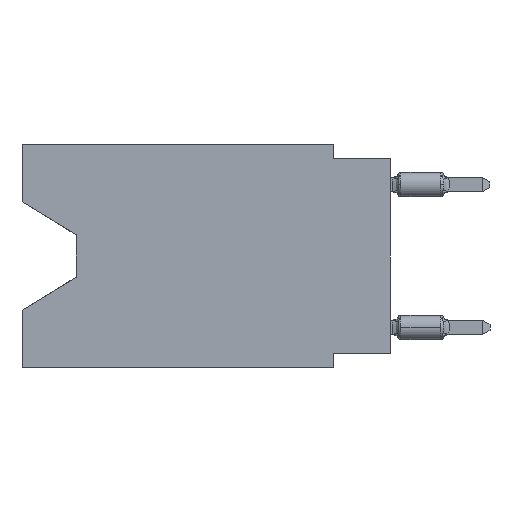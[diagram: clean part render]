
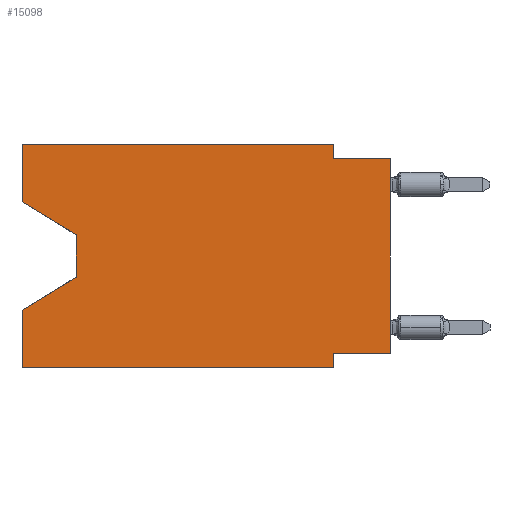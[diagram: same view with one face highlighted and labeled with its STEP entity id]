
A CAD part, left-side view. The second image highlights one B-rep face of the part: STEP entity #15098.
In plain terms, the highlighted planar face has unit normal (-1, 0, 0).
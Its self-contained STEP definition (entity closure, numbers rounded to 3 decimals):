
#19 = CARTESIAN_POINT ( 'NONE',  ( 0., 0., 0. ) ) ;
#44 = EDGE_LOOP ( 'NONE', ( #9401, #10544, #11426, #8220, #8632, #4534, #13998, #9303, #6205, #1182, #1276, #12741 ) ) ;
#261 = CARTESIAN_POINT ( 'NONE',  ( 0., 16.383, -7.36 ) ) ;
#678 = EDGE_CURVE ( 'NONE', #10650, #6573, #16260, .T. ) ;
#911 = VECTOR ( 'NONE', #5803, 1000. ) ;
#1005 = DIRECTION ( 'NONE',  ( 0., 0., -1. ) ) ;
#1182 = ORIENTED_EDGE ( 'NONE', *, *, #10891, .F. ) ;
#1225 = AXIS2_PLACEMENT_3D ( 'NONE', #1254, #7778, #1005 ) ;
#1254 = CARTESIAN_POINT ( 'NONE',  ( 0., 16.383, 0. ) ) ;
#1276 = ORIENTED_EDGE ( 'NONE', *, *, #12093, .F. ) ;
#1314 = CARTESIAN_POINT ( 'NONE',  ( 0., 16.383, 0. ) ) ;
#1611 = LINE ( 'NONE', #9928, #1913 ) ;
#1913 = VECTOR ( 'NONE', #12980, 1000. ) ;
#2863 = VECTOR ( 'NONE', #7139, 1000. ) ;
#2887 = VERTEX_POINT ( 'NONE', #13137 ) ;
#2916 = VECTOR ( 'NONE', #14248, 1000. ) ;
#4529 = CARTESIAN_POINT ( 'NONE',  ( 0., 2.54, 0. ) ) ;
#4534 = ORIENTED_EDGE ( 'NONE', *, *, #13500, .F. ) ;
#5208 = CARTESIAN_POINT ( 'NONE',  ( 0., 16.383, 0. ) ) ;
#5517 = VERTEX_POINT ( 'NONE', #261 ) ;
#5581 = CARTESIAN_POINT ( 'NONE',  ( 0., 16.383, -2.546 ) ) ;
#5620 = DIRECTION ( 'NONE',  ( 0., 0., -1. ) ) ;
#5654 = CARTESIAN_POINT ( 'NONE',  ( 0., 2.54, -9.271 ) ) ;
#5803 = DIRECTION ( 'NONE',  ( 0., 1., 0. ) ) ;
#5956 = VECTOR ( 'NONE', #5620, 1000. ) ;
#5979 = CARTESIAN_POINT ( 'NONE',  ( 0., 16.383, -2.546 ) ) ;
#6205 = ORIENTED_EDGE ( 'NONE', *, *, #11991, .F. ) ;
#6573 = VERTEX_POINT ( 'NONE', #11096 ) ;
#6591 = DIRECTION ( 'NONE',  ( 0., 0., -1. ) ) ;
#6621 = DIRECTION ( 'NONE',  ( 0., -1., 0. ) ) ;
#6687 = LINE ( 'NONE', #12307, #15581 ) ;
#7030 = CARTESIAN_POINT ( 'NONE',  ( 0., 0., -9.271 ) ) ;
#7057 = VECTOR ( 'NONE', #14948, 1000. ) ;
#7139 = DIRECTION ( 'NONE',  ( 0., 0., -1. ) ) ;
#7435 = VERTEX_POINT ( 'NONE', #4529 ) ;
#7647 = CARTESIAN_POINT ( 'NONE',  ( 0., 16.383, -9.906 ) ) ;
#7697 = VECTOR ( 'NONE', #13743, 1000. ) ;
#7778 = DIRECTION ( 'NONE',  ( 1., 0., 0. ) ) ;
#8040 = PLANE ( 'NONE',  #1225 ) ;
#8220 = ORIENTED_EDGE ( 'NONE', *, *, #9516, .F. ) ;
#8400 = VERTEX_POINT ( 'NONE', #12094 ) ;
#8482 = DIRECTION ( 'NONE',  ( 0., -0.855, -0.519 ) ) ;
#8632 = ORIENTED_EDGE ( 'NONE', *, *, #10677, .T. ) ;
#8814 = VECTOR ( 'NONE', #6621, 1000. ) ;
#9027 = CARTESIAN_POINT ( 'NONE',  ( 0., 2.54, -0.635 ) ) ;
#9072 = LINE ( 'NONE', #5208, #11628 ) ;
#9150 = LINE ( 'NONE', #7647, #2916 ) ;
#9303 = ORIENTED_EDGE ( 'NONE', *, *, #16847, .T. ) ;
#9354 = VECTOR ( 'NONE', #8482, 1000. ) ;
#9401 = ORIENTED_EDGE ( 'NONE', *, *, #13070, .T. ) ;
#9516 = EDGE_CURVE ( 'NONE', #12317, #5517, #1611, .T. ) ;
#9762 = CARTESIAN_POINT ( 'NONE',  ( 0., 13.97, -4.013 ) ) ;
#9928 = CARTESIAN_POINT ( 'NONE',  ( 0., 16.383, 0. ) ) ;
#10223 = LINE ( 'NONE', #11801, #8814 ) ;
#10544 = ORIENTED_EDGE ( 'NONE', *, *, #13833, .T. ) ;
#10650 = VERTEX_POINT ( 'NONE', #5979 ) ;
#10677 = EDGE_CURVE ( 'NONE', #12317, #8400, #9150, .T. ) ;
#10820 = VECTOR ( 'NONE', #13360, 1000. ) ;
#10891 = EDGE_CURVE ( 'NONE', #7435, #12380, #6687, .T. ) ;
#11096 = CARTESIAN_POINT ( 'NONE',  ( 0., 16.383, 0. ) ) ;
#11426 = ORIENTED_EDGE ( 'NONE', *, *, #15208, .T. ) ;
#11628 = VECTOR ( 'NONE', #14438, 1000. ) ;
#11801 = CARTESIAN_POINT ( 'NONE',  ( 0., 0., -0.635 ) ) ;
#11851 = VERTEX_POINT ( 'NONE', #5654 ) ;
#11991 = EDGE_CURVE ( 'NONE', #12380, #16071, #10223, .T. ) ;
#12093 = EDGE_CURVE ( 'NONE', #6573, #7435, #9072, .T. ) ;
#12094 = CARTESIAN_POINT ( 'NONE',  ( 0., 2.54, -9.906 ) ) ;
#12207 = CARTESIAN_POINT ( 'NONE',  ( 0., 0., -0.635 ) ) ;
#12307 = CARTESIAN_POINT ( 'NONE',  ( 0., 2.54, 0. ) ) ;
#12317 = VERTEX_POINT ( 'NONE', #12585 ) ;
#12336 = CARTESIAN_POINT ( 'NONE',  ( 0., 13.97, -5.893 ) ) ;
#12380 = VERTEX_POINT ( 'NONE', #9027 ) ;
#12414 = LINE ( 'NONE', #13569, #7697 ) ;
#12480 = LINE ( 'NONE', #7030, #911 ) ;
#12585 = CARTESIAN_POINT ( 'NONE',  ( 0., 16.383, -9.906 ) ) ;
#12741 = ORIENTED_EDGE ( 'NONE', *, *, #678, .F. ) ;
#12980 = DIRECTION ( 'NONE',  ( 0., 0., 1. ) ) ;
#13070 = EDGE_CURVE ( 'NONE', #10650, #15664, #15152, .T. ) ;
#13137 = CARTESIAN_POINT ( 'NONE',  ( 0., 0., -9.271 ) ) ;
#13360 = DIRECTION ( 'NONE',  ( 0., 0., 1. ) ) ;
#13479 = VERTEX_POINT ( 'NONE', #12336 ) ;
#13500 = EDGE_CURVE ( 'NONE', #11851, #8400, #15215, .T. ) ;
#13548 = LINE ( 'NONE', #19, #7057 ) ;
#13569 = CARTESIAN_POINT ( 'NONE',  ( 0., 13.97, -5.893 ) ) ;
#13743 = DIRECTION ( 'NONE',  ( 0., 0.855, -0.519 ) ) ;
#13833 = EDGE_CURVE ( 'NONE', #15664, #13479, #14942, .T. ) ;
#13848 = EDGE_CURVE ( 'NONE', #2887, #11851, #12480, .T. ) ;
#13998 = ORIENTED_EDGE ( 'NONE', *, *, #13848, .F. ) ;
#14248 = DIRECTION ( 'NONE',  ( 0., -1., 0. ) ) ;
#14438 = DIRECTION ( 'NONE',  ( 0., -1., 0. ) ) ;
#14942 = LINE ( 'NONE', #9762, #5956 ) ;
#14948 = DIRECTION ( 'NONE',  ( 0., 0., 1. ) ) ;
#15098 = ADVANCED_FACE ( 'NONE', ( #15678 ), #8040, .F. ) ;
#15152 = LINE ( 'NONE', #5581, #9354 ) ;
#15208 = EDGE_CURVE ( 'NONE', #13479, #5517, #12414, .T. ) ;
#15215 = LINE ( 'NONE', #16471, #2863 ) ;
#15581 = VECTOR ( 'NONE', #6591, 1000. ) ;
#15664 = VERTEX_POINT ( 'NONE', #16089 ) ;
#15678 = FACE_OUTER_BOUND ( 'NONE', #44, .T. ) ;
#16071 = VERTEX_POINT ( 'NONE', #12207 ) ;
#16089 = CARTESIAN_POINT ( 'NONE',  ( 0., 13.97, -4.013 ) ) ;
#16260 = LINE ( 'NONE', #1314, #10820 ) ;
#16471 = CARTESIAN_POINT ( 'NONE',  ( 0., 2.54, -9.906 ) ) ;
#16847 = EDGE_CURVE ( 'NONE', #2887, #16071, #13548, .T. ) ;
